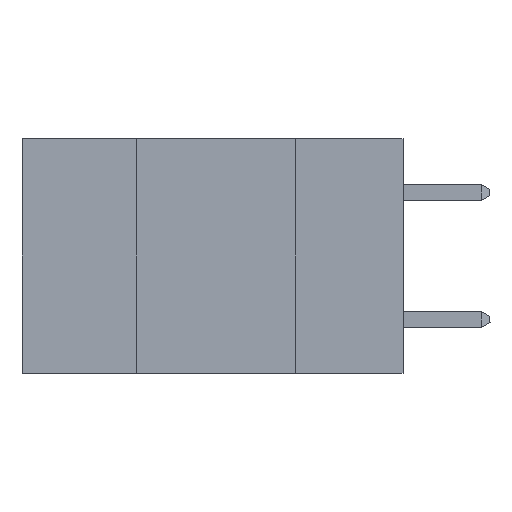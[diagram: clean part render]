
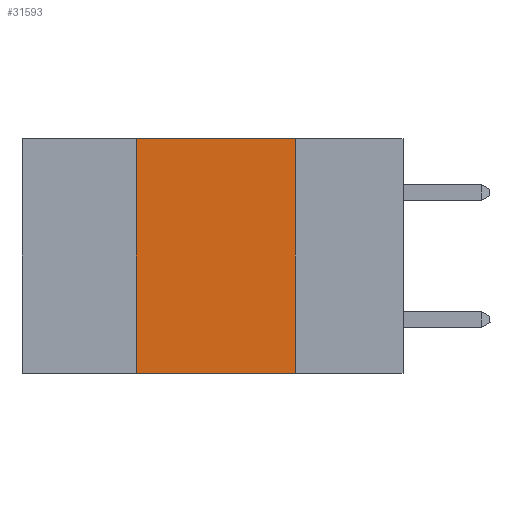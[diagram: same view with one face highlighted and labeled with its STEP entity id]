
A CAD part, left-side view. The second image highlights one B-rep face of the part: STEP entity #31593.
In plain terms, the highlighted planar face has unit normal (-1, 0, 0).
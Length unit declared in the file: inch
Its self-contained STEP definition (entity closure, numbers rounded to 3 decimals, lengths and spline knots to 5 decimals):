
#1176 = CARTESIAN_POINT ( 'NONE',  ( 0., 0.42, 0. ) ) ;
#2611 = DIRECTION ( 'NONE',  ( 0., 0., -1. ) ) ;
#4107 = CARTESIAN_POINT ( 'NONE',  ( 0., 0.42, 0. ) ) ;
#4779 = VERTEX_POINT ( 'NONE', #21919 ) ;
#7443 = VECTOR ( 'NONE', #8101, 39.37008 ) ;
#8101 = DIRECTION ( 'NONE',  ( 0., -1., 0. ) ) ;
#8213 = CARTESIAN_POINT ( 'NONE',  ( 0., 0.6, 0. ) ) ;
#13407 = CARTESIAN_POINT ( 'NONE',  ( 0., 0.17, 0. ) ) ;
#14868 = EDGE_CURVE ( 'NONE', #30890, #4779, #31246, .T. ) ;
#18000 = ORIENTED_EDGE ( 'NONE', *, *, #26725, .T. ) ;
#19752 = EDGE_CURVE ( 'NONE', #4779, #31523, #36107, .T. ) ;
#19904 = EDGE_LOOP ( 'NONE', ( #32151, #24316, #25489, #18000 ) ) ;
#21470 = VECTOR ( 'NONE', #29960, 39.37008 ) ;
#21471 = EDGE_CURVE ( 'NONE', #29614, #30890, #29613, .T. ) ;
#21919 = CARTESIAN_POINT ( 'NONE',  ( 0., 0.17, 0. ) ) ;
#22513 = CARTESIAN_POINT ( 'NONE',  ( 0., 0.6, 0. ) ) ;
#22557 = DIRECTION ( 'NONE',  ( 1., 0., 0. ) ) ;
#24316 = ORIENTED_EDGE ( 'NONE', *, *, #14868, .F. ) ;
#25236 = CARTESIAN_POINT ( 'NONE',  ( 0., 0.6, -0.37 ) ) ;
#25489 = ORIENTED_EDGE ( 'NONE', *, *, #21471, .F. ) ;
#25531 = PLANE ( 'NONE',  #36143 ) ;
#25604 = LINE ( 'NONE', #25236, #7443 ) ;
#26532 = CARTESIAN_POINT ( 'NONE',  ( 0., 0.42, -0.37 ) ) ;
#26725 = EDGE_CURVE ( 'NONE', #29614, #31523, #25604, .T. ) ;
#26830 = DIRECTION ( 'NONE',  ( 0., 0., 1. ) ) ;
#28680 = CARTESIAN_POINT ( 'NONE',  ( 0., 0.17, -0.37 ) ) ;
#29613 = LINE ( 'NONE', #4107, #32832 ) ;
#29614 = VERTEX_POINT ( 'NONE', #26532 ) ;
#29960 = DIRECTION ( 'NONE',  ( 0., 0., -1. ) ) ;
#30205 = VECTOR ( 'NONE', #36461, 39.37008 ) ;
#30890 = VERTEX_POINT ( 'NONE', #1176 ) ;
#31246 = LINE ( 'NONE', #22513, #30205 ) ;
#31523 = VERTEX_POINT ( 'NONE', #28680 ) ;
#31593 = ADVANCED_FACE ( 'NONE', ( #34269 ), #25531, .F. ) ;
#32151 = ORIENTED_EDGE ( 'NONE', *, *, #19752, .F. ) ;
#32832 = VECTOR ( 'NONE', #26830, 39.37008 ) ;
#34269 = FACE_OUTER_BOUND ( 'NONE', #19904, .T. ) ;
#36107 = LINE ( 'NONE', #13407, #21470 ) ;
#36143 = AXIS2_PLACEMENT_3D ( 'NONE', #8213, #22557, #2611 ) ;
#36461 = DIRECTION ( 'NONE',  ( 0., -1., 0. ) ) ;
